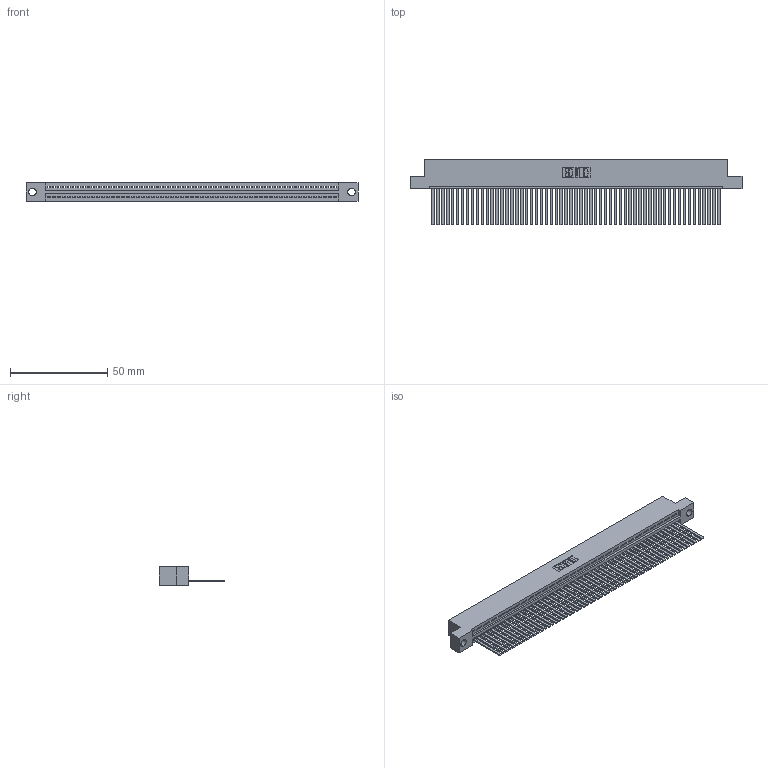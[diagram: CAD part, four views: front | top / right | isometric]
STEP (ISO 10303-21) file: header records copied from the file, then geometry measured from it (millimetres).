
FILE_DESCRIPTION (( 'STEP AP203' ), '1' );
FILE_NAME ('345-059-544-104.STEP', '2019-10-10T20:41:40', ( '' ), ( '' ), 'SwSTEP 2.0', 'SolidWorks 2016', '' );
FILE_SCHEMA (( 'CONFIG_CONTROL_DESIGN' ));
Length unit declared in the file: inch
Products named in the file (3): 345-292-001_345-293-144; 345-059-544-104; 345 Part_Flush Mounting Lugs - 0.156 Dia-TH
Assembly tree (60 placements, depth 2):
  345-059-544-104
    345 Part_Flush Mounting Lugs - 0.156 Dia-TH
    345-292-001_345-293-144  x59
Bounding box: 171.07 x 33.96 x 9.4 mm (x, y, z)
Volume: 16983 mm3; surface area: 24660 mm2
Topology: 60 solids, 60 shells, 3194 faces, 9663 edges, 6362 vertices
Faces by surface type: plane 2204, cylinder 990
Entity records: 41935 total; most frequent: CARTESIAN_POINT 7269, ORIENTED_EDGE 7262, DIRECTION 6321, EDGE_CURVE 3631, VECTOR 3267, LINE 3267, VERTEX_POINT 2418, AXIS2_PLACEMENT_3D 1527
